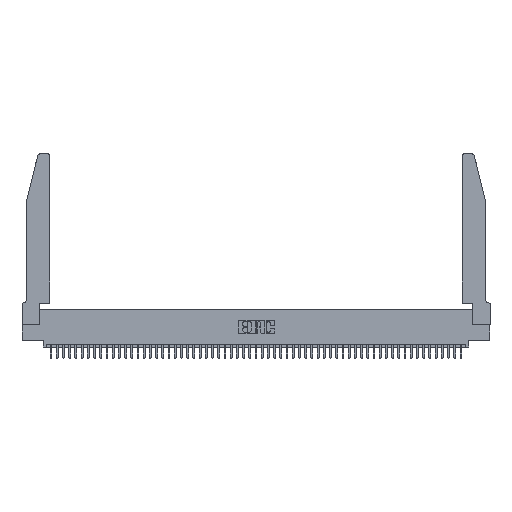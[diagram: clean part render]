
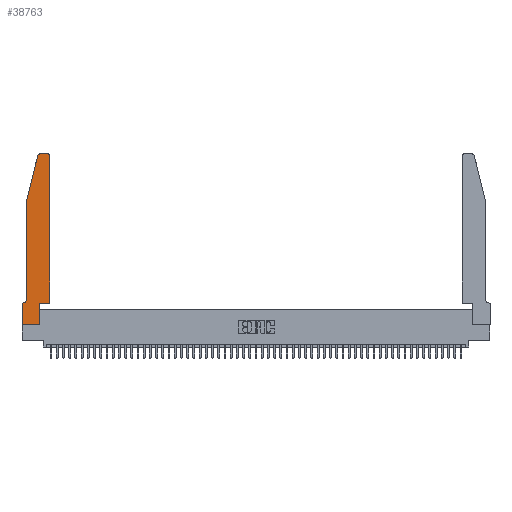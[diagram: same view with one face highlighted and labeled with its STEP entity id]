
A CAD part, top view. The second image highlights one B-rep face of the part: STEP entity #38763.
In plain terms, the highlighted planar face has unit normal (0, 0, 1).
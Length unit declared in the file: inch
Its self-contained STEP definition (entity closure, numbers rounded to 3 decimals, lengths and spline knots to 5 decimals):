
#243 = VECTOR ( 'NONE', #45425, 39.37008 ) ;
#433 = CARTESIAN_POINT ( 'NONE',  ( 0.4505, 0.35, 0.37 ) ) ;
#500 = VERTEX_POINT ( 'NONE', #37715 ) ;
#1540 = DIRECTION ( 'NONE',  ( 1., 0., 0. ) ) ;
#2201 = ORIENTED_EDGE ( 'NONE', *, *, #15825, .T. ) ;
#2382 = LINE ( 'NONE', #4903, #24665 ) ;
#2921 = DIRECTION ( 'NONE',  ( -1., 0., 0. ) ) ;
#3117 = EDGE_CURVE ( 'NONE', #46921, #37846, #40879, .T. ) ;
#4903 = CARTESIAN_POINT ( 'NONE',  ( 0.0755, 2., 0.37 ) ) ;
#5205 = EDGE_CURVE ( 'NONE', #500, #44611, #34043, .T. ) ;
#5579 = CARTESIAN_POINT ( 'NONE',  ( 0.0755, 0.42, 0.37 ) ) ;
#6039 = LINE ( 'NONE', #26627, #29618 ) ;
#6206 = VERTEX_POINT ( 'NONE', #22910 ) ;
#6703 = EDGE_CURVE ( 'NONE', #37846, #29606, #2382, .T. ) ;
#7196 = VERTEX_POINT ( 'NONE', #40916 ) ;
#7638 = VECTOR ( 'NONE', #24082, 39.37008 ) ;
#8414 = EDGE_CURVE ( 'NONE', #7196, #500, #12830, .T. ) ;
#8781 = CARTESIAN_POINT ( 'NONE',  ( 0.2865, 0.35, 0.37 ) ) ;
#9341 = VECTOR ( 'NONE', #38185, 39.37008 ) ;
#9370 = VECTOR ( 'NONE', #24259, 39.37008 ) ;
#9513 = DIRECTION ( 'NONE',  ( 0., 0., 1. ) ) ;
#11405 = ORIENTED_EDGE ( 'NONE', *, *, #34137, .T. ) ;
#11636 = CARTESIAN_POINT ( 'NONE',  ( 0.2605, 2.75, 0.37 ) ) ;
#11939 = CARTESIAN_POINT ( 'NONE',  ( 0.0755, 2., 0.37 ) ) ;
#12175 = ORIENTED_EDGE ( 'NONE', *, *, #17069, .T. ) ;
#12180 = ORIENTED_EDGE ( 'NONE', *, *, #3117, .T. ) ;
#12761 = ORIENTED_EDGE ( 'NONE', *, *, #33158, .T. ) ;
#12830 = LINE ( 'NONE', #15424, #22646 ) ;
#13027 = ORIENTED_EDGE ( 'NONE', *, *, #8414, .T. ) ;
#13752 = EDGE_CURVE ( 'NONE', #6206, #18412, #53477, .T. ) ;
#14362 = FACE_OUTER_BOUND ( 'NONE', #26155, .T. ) ;
#15424 = CARTESIAN_POINT ( 'NONE',  ( 0.0755, 0.35, 0.37 ) ) ;
#15591 = EDGE_CURVE ( 'NONE', #46127, #7196, #43453, .T. ) ;
#15825 = EDGE_CURVE ( 'NONE', #21489, #6206, #19201, .T. ) ;
#16529 = CARTESIAN_POINT ( 'NONE',  ( 0.4205, 2.72, 0.37 ) ) ;
#17069 = EDGE_CURVE ( 'NONE', #32822, #38366, #22988, .T. ) ;
#18175 = CARTESIAN_POINT ( 'NONE',  ( 0., 0.35, 0.37 ) ) ;
#18412 = VERTEX_POINT ( 'NONE', #50096 ) ;
#19068 = CARTESIAN_POINT ( 'NONE',  ( 0.284, 2.75, 0.37 ) ) ;
#19201 = LINE ( 'NONE', #8781, #40141 ) ;
#19217 = CARTESIAN_POINT ( 'NONE',  ( 0.0055, 0.42, 0.37 ) ) ;
#19530 = CARTESIAN_POINT ( 'NONE',  ( 0., 0., 0.37 ) ) ;
#20012 = ORIENTED_EDGE ( 'NONE', *, *, #6703, .T. ) ;
#20735 = DIRECTION ( 'NONE',  ( 1., 0., 0. ) ) ;
#21489 = VERTEX_POINT ( 'NONE', #46147 ) ;
#21511 = ORIENTED_EDGE ( 'NONE', *, *, #27228, .T. ) ;
#21632 = VECTOR ( 'NONE', #32123, 39.37008 ) ;
#22407 = DIRECTION ( 'NONE',  ( 0., 0., 1. ) ) ;
#22646 = VECTOR ( 'NONE', #2921, 39.37008 ) ;
#22910 = CARTESIAN_POINT ( 'NONE',  ( 0.2865, 0.35, 0.37 ) ) ;
#22988 = CIRCLE ( 'NONE', #51566, 0.03 ) ;
#23423 = DIRECTION ( 'NONE',  ( -1., 0., 0. ) ) ;
#24082 = DIRECTION ( 'NONE',  ( 1., 0., 0. ) ) ;
#24259 = DIRECTION ( 'NONE',  ( -1., 0., 0. ) ) ;
#24665 = VECTOR ( 'NONE', #34174, 39.37008 ) ;
#26035 = CARTESIAN_POINT ( 'NONE',  ( 0.4505, 2.72, 0.37 ) ) ;
#26155 = EDGE_LOOP ( 'NONE', ( #53473, #12180, #20012, #12761, #29040, #13027, #43724, #11405, #2201, #31613, #21511, #12175 ) ) ;
#26627 = CARTESIAN_POINT ( 'NONE',  ( 0., 0., 0.37 ) ) ;
#27228 = EDGE_CURVE ( 'NONE', #18412, #32822, #32893, .T. ) ;
#28278 = CARTESIAN_POINT ( 'NONE',  ( 0.4205, 2.75, 0.37 ) ) ;
#29040 = ORIENTED_EDGE ( 'NONE', *, *, #15591, .T. ) ;
#29606 = VERTEX_POINT ( 'NONE', #29949 ) ;
#29618 = VECTOR ( 'NONE', #1540, 39.37008 ) ;
#29949 = CARTESIAN_POINT ( 'NONE',  ( 0.0755, 2., 0.37 ) ) ;
#31613 = ORIENTED_EDGE ( 'NONE', *, *, #13752, .T. ) ;
#32123 = DIRECTION ( 'NONE',  ( 0., -1., 0. ) ) ;
#32351 = LINE ( 'NONE', #11939, #243 ) ;
#32822 = VERTEX_POINT ( 'NONE', #26035 ) ;
#32893 = LINE ( 'NONE', #433, #9341 ) ;
#33158 = EDGE_CURVE ( 'NONE', #29606, #46127, #32351, .T. ) ;
#33523 = CARTESIAN_POINT ( 'NONE',  ( 0., 0., 0.37 ) ) ;
#34043 = LINE ( 'NONE', #19530, #21632 ) ;
#34137 = EDGE_CURVE ( 'NONE', #44611, #21489, #6039, .T. ) ;
#34174 = DIRECTION ( 'NONE',  ( -0.239, -0.971, 0. ) ) ;
#34555 = CARTESIAN_POINT ( 'NONE',  ( 0.284, 2.72, 0.37 ) ) ;
#36727 = CARTESIAN_POINT ( 'NONE',  ( 0.4505, 0.35, 0.37 ) ) ;
#37715 = CARTESIAN_POINT ( 'NONE',  ( 0., 0.35, 0.37 ) ) ;
#37846 = VERTEX_POINT ( 'NONE', #43672 ) ;
#38180 = AXIS2_PLACEMENT_3D ( 'NONE', #34555, #9513, #38777 ) ;
#38185 = DIRECTION ( 'NONE',  ( 0., 1., 0. ) ) ;
#38366 = VERTEX_POINT ( 'NONE', #28278 ) ;
#38763 = ADVANCED_FACE ( 'NONE', ( #14362 ), #43255, .T. ) ;
#38777 = DIRECTION ( 'NONE',  ( 1., 0., 0. ) ) ;
#40141 = VECTOR ( 'NONE', #50669, 39.37008 ) ;
#40879 = CIRCLE ( 'NONE', #38180, 0.03 ) ;
#40916 = CARTESIAN_POINT ( 'NONE',  ( 0.0055, 0.35, 0.37 ) ) ;
#43255 = PLANE ( 'NONE',  #53970 ) ;
#43453 = CIRCLE ( 'NONE', #50114, 0.07 ) ;
#43672 = CARTESIAN_POINT ( 'NONE',  ( 0.25487, 2.72718, 0.37 ) ) ;
#43724 = ORIENTED_EDGE ( 'NONE', *, *, #5205, .T. ) ;
#44457 = EDGE_CURVE ( 'NONE', #38366, #46921, #44557, .T. ) ;
#44557 = LINE ( 'NONE', #11636, #9370 ) ;
#44611 = VERTEX_POINT ( 'NONE', #33523 ) ;
#45425 = DIRECTION ( 'NONE',  ( 0., -1., 0. ) ) ;
#45807 = DIRECTION ( 'NONE',  ( 0., 0., 1. ) ) ;
#46127 = VERTEX_POINT ( 'NONE', #5579 ) ;
#46147 = CARTESIAN_POINT ( 'NONE',  ( 0.2865, 0., 0.37 ) ) ;
#46921 = VERTEX_POINT ( 'NONE', #19068 ) ;
#48498 = DIRECTION ( 'NONE',  ( 0., 0., -1. ) ) ;
#50096 = CARTESIAN_POINT ( 'NONE',  ( 0.4505, 0.35, 0.37 ) ) ;
#50114 = AXIS2_PLACEMENT_3D ( 'NONE', #19217, #48498, #23423 ) ;
#50669 = DIRECTION ( 'NONE',  ( 0., 1., 0. ) ) ;
#51566 = AXIS2_PLACEMENT_3D ( 'NONE', #16529, #45807, #20735 ) ;
#51672 = DIRECTION ( 'NONE',  ( 1., 0., 0. ) ) ;
#53473 = ORIENTED_EDGE ( 'NONE', *, *, #44457, .T. ) ;
#53477 = LINE ( 'NONE', #36727, #7638 ) ;
#53970 = AXIS2_PLACEMENT_3D ( 'NONE', #18175, #22407, #51672 ) ;
